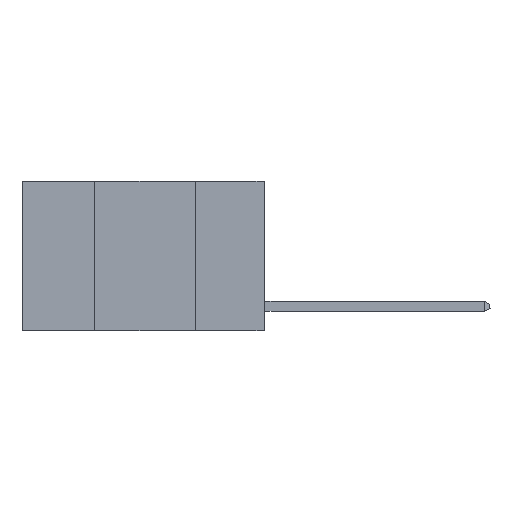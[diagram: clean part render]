
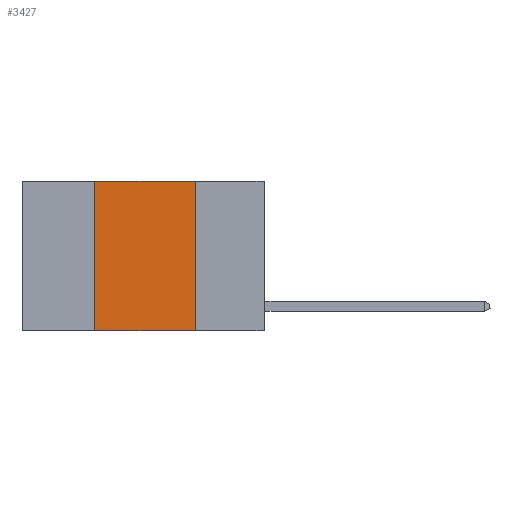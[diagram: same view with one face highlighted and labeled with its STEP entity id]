
A CAD part, left-side view. The second image highlights one B-rep face of the part: STEP entity #3427.
In plain terms, the highlighted planar face has unit normal (-1, 0, 0).
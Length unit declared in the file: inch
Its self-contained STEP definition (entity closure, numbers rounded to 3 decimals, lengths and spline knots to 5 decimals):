
#204 = DIRECTION ( 'NONE',  ( 0., -1., 0. ) ) ;
#971 = DIRECTION ( 'NONE',  ( 0., 0., -1. ) ) ;
#1744 = VERTEX_POINT ( 'NONE', #15164 ) ;
#2026 = DIRECTION ( 'NONE',  ( 0., 0., -1. ) ) ;
#2396 = CARTESIAN_POINT ( 'NONE',  ( 0., 0.6, 0. ) ) ;
#2549 = LINE ( 'NONE', #2396, #8922 ) ;
#2616 = AXIS2_PLACEMENT_3D ( 'NONE', #7916, #5800, #971 ) ;
#3022 = LINE ( 'NONE', #11110, #8885 ) ;
#3427 = ADVANCED_FACE ( 'NONE', ( #14108 ), #9395, .F. ) ;
#3769 = EDGE_CURVE ( 'NONE', #1744, #8982, #5402, .T. ) ;
#4350 = DIRECTION ( 'NONE',  ( 0., -1., 0. ) ) ;
#4376 = ORIENTED_EDGE ( 'NONE', *, *, #12606, .F. ) ;
#4940 = CARTESIAN_POINT ( 'NONE',  ( 0., 0.17, -0.37 ) ) ;
#5137 = ORIENTED_EDGE ( 'NONE', *, *, #3769, .F. ) ;
#5402 = LINE ( 'NONE', #8677, #9114 ) ;
#5709 = VECTOR ( 'NONE', #2026, 39.37008 ) ;
#5800 = DIRECTION ( 'NONE',  ( 1., 0., 0. ) ) ;
#5940 = CARTESIAN_POINT ( 'NONE',  ( 0., 0.42, 0. ) ) ;
#6613 = CARTESIAN_POINT ( 'NONE',  ( 0., 0.17, 0. ) ) ;
#6901 = EDGE_CURVE ( 'NONE', #1744, #12465, #3022, .T. ) ;
#7916 = CARTESIAN_POINT ( 'NONE',  ( 0., 0.6, 0. ) ) ;
#8677 = CARTESIAN_POINT ( 'NONE',  ( 0., 0.42, 0. ) ) ;
#8885 = VECTOR ( 'NONE', #4350, 39.37008 ) ;
#8922 = VECTOR ( 'NONE', #204, 39.37008 ) ;
#8982 = VERTEX_POINT ( 'NONE', #5940 ) ;
#9114 = VECTOR ( 'NONE', #10022, 39.37008 ) ;
#9150 = VERTEX_POINT ( 'NONE', #13840 ) ;
#9395 = PLANE ( 'NONE',  #2616 ) ;
#10022 = DIRECTION ( 'NONE',  ( 0., 0., 1. ) ) ;
#10097 = ORIENTED_EDGE ( 'NONE', *, *, #6901, .T. ) ;
#11110 = CARTESIAN_POINT ( 'NONE',  ( 0., 0.6, -0.37 ) ) ;
#12465 = VERTEX_POINT ( 'NONE', #4940 ) ;
#12606 = EDGE_CURVE ( 'NONE', #9150, #12465, #14854, .T. ) ;
#13075 = EDGE_LOOP ( 'NONE', ( #4376, #14882, #5137, #10097 ) ) ;
#13225 = EDGE_CURVE ( 'NONE', #8982, #9150, #2549, .T. ) ;
#13840 = CARTESIAN_POINT ( 'NONE',  ( 0., 0.17, 0. ) ) ;
#14108 = FACE_OUTER_BOUND ( 'NONE', #13075, .T. ) ;
#14854 = LINE ( 'NONE', #6613, #5709 ) ;
#14882 = ORIENTED_EDGE ( 'NONE', *, *, #13225, .F. ) ;
#15164 = CARTESIAN_POINT ( 'NONE',  ( 0., 0.42, -0.37 ) ) ;
